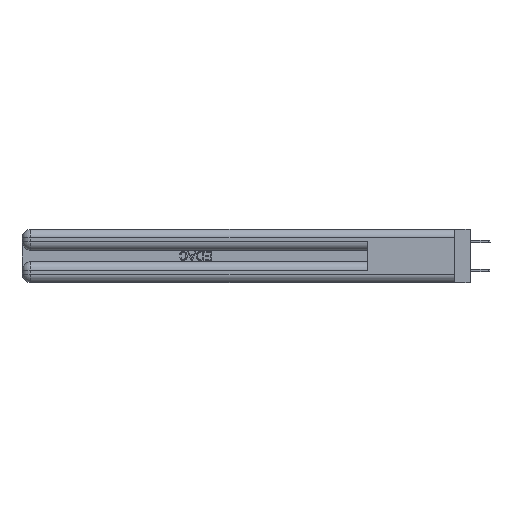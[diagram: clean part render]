
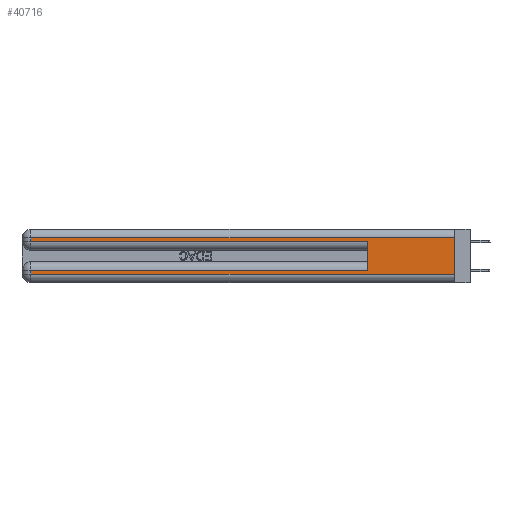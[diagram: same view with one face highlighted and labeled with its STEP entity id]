
A CAD part, left-side view. The second image highlights one B-rep face of the part: STEP entity #40716.
In plain terms, the highlighted planar face has unit normal (-1, 0, 0).
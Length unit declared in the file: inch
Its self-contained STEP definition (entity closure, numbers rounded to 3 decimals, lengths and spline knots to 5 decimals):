
#1308 = CARTESIAN_POINT ( 'NONE',  ( 0., 0., 0.37 ) ) ;
#1571 = DIRECTION ( 'NONE',  ( 0., -1., 0. ) ) ;
#2276 = AXIS2_PLACEMENT_3D ( 'NONE', #1308, #15779, #30198 ) ;
#2425 = VERTEX_POINT ( 'NONE', #5387 ) ;
#2899 = VERTEX_POINT ( 'NONE', #8666 ) ;
#4686 = VECTOR ( 'NONE', #23078, 39.37008 ) ;
#5306 = CARTESIAN_POINT ( 'NONE',  ( 0., 0.6, 0.085 ) ) ;
#5387 = CARTESIAN_POINT ( 'NONE',  ( 0., 2.94, 0.06 ) ) ;
#5488 = VECTOR ( 'NONE', #1571, 39.37008 ) ;
#7298 = EDGE_CURVE ( 'NONE', #46163, #21955, #8669, .T. ) ;
#7451 = EDGE_CURVE ( 'NONE', #21955, #2425, #9376, .T. ) ;
#8666 = CARTESIAN_POINT ( 'NONE',  ( 0., 2.94, 0.31 ) ) ;
#8669 = LINE ( 'NONE', #41094, #4686 ) ;
#9069 = DIRECTION ( 'NONE',  ( 0., 0., -1. ) ) ;
#9376 = LINE ( 'NONE', #13370, #44769 ) ;
#9484 = ORIENTED_EDGE ( 'NONE', *, *, #7298, .T. ) ;
#11022 = LINE ( 'NONE', #29865, #19572 ) ;
#11464 = DIRECTION ( 'NONE',  ( 0., -1., 0. ) ) ;
#12067 = CARTESIAN_POINT ( 'NONE',  ( 0., 0., 0.06 ) ) ;
#12344 = ORIENTED_EDGE ( 'NONE', *, *, #45141, .T. ) ;
#12583 = DIRECTION ( 'NONE',  ( 0., 1., 0. ) ) ;
#13263 = VERTEX_POINT ( 'NONE', #26310 ) ;
#13370 = CARTESIAN_POINT ( 'NONE',  ( 0., 2.94, 0.37 ) ) ;
#15779 = DIRECTION ( 'NONE',  ( 1., 0., 0. ) ) ;
#15793 = ORIENTED_EDGE ( 'NONE', *, *, #34491, .T. ) ;
#15811 = CARTESIAN_POINT ( 'NONE',  ( 0., 0.6, 0.145 ) ) ;
#16283 = DIRECTION ( 'NONE',  ( 0., 0., 1. ) ) ;
#16447 = DIRECTION ( 'NONE',  ( 0., 0., -1. ) ) ;
#19075 = ORIENTED_EDGE ( 'NONE', *, *, #24551, .F. ) ;
#19327 = FACE_OUTER_BOUND ( 'NONE', #39699, .T. ) ;
#19572 = VECTOR ( 'NONE', #29424, 39.37008 ) ;
#20062 = CARTESIAN_POINT ( 'NONE',  ( 0., 2.94, 0.085 ) ) ;
#21001 = VECTOR ( 'NONE', #12583, 39.37008 ) ;
#21955 = VERTEX_POINT ( 'NONE', #20062 ) ;
#22967 = VECTOR ( 'NONE', #11464, 39.37008 ) ;
#23078 = DIRECTION ( 'NONE',  ( 0., 1., 0. ) ) ;
#24154 = ORIENTED_EDGE ( 'NONE', *, *, #37795, .T. ) ;
#24551 = EDGE_CURVE ( 'NONE', #46163, #13263, #27652, .T. ) ;
#24935 = CARTESIAN_POINT ( 'NONE',  ( 0., 2.94, 0.285 ) ) ;
#25213 = VERTEX_POINT ( 'NONE', #24935 ) ;
#26141 = CARTESIAN_POINT ( 'NONE',  ( 0., 0., 0.06 ) ) ;
#26310 = CARTESIAN_POINT ( 'NONE',  ( 0., 0.6, 0.285 ) ) ;
#26341 = CARTESIAN_POINT ( 'NONE',  ( 0., 2.94, 0.37 ) ) ;
#27261 = LINE ( 'NONE', #26341, #36310 ) ;
#27652 = LINE ( 'NONE', #15811, #38621 ) ;
#29424 = DIRECTION ( 'NONE',  ( 0., 0., -1. ) ) ;
#29865 = CARTESIAN_POINT ( 'NONE',  ( 0., 0., 0.37 ) ) ;
#30198 = DIRECTION ( 'NONE',  ( 0., 0., -1. ) ) ;
#31731 = ORIENTED_EDGE ( 'NONE', *, *, #39120, .F. ) ;
#32503 = CARTESIAN_POINT ( 'NONE',  ( 0., 0., 0.285 ) ) ;
#32550 = VERTEX_POINT ( 'NONE', #26141 ) ;
#33764 = PLANE ( 'NONE',  #2276 ) ;
#34491 = EDGE_CURVE ( 'NONE', #39232, #2899, #38134, .T. ) ;
#36310 = VECTOR ( 'NONE', #9069, 39.37008 ) ;
#36511 = LINE ( 'NONE', #32503, #22967 ) ;
#37795 = EDGE_CURVE ( 'NONE', #2899, #25213, #27261, .T. ) ;
#38134 = LINE ( 'NONE', #45959, #21001 ) ;
#38621 = VECTOR ( 'NONE', #16283, 39.37008 ) ;
#39120 = EDGE_CURVE ( 'NONE', #39232, #32550, #11022, .T. ) ;
#39232 = VERTEX_POINT ( 'NONE', #41033 ) ;
#39699 = EDGE_LOOP ( 'NONE', ( #31731, #15793, #24154, #43012, #19075, #9484, #43278, #12344 ) ) ;
#40716 = ADVANCED_FACE ( 'NONE', ( #19327 ), #33764, .F. ) ;
#41033 = CARTESIAN_POINT ( 'NONE',  ( 0., 0., 0.31 ) ) ;
#41094 = CARTESIAN_POINT ( 'NONE',  ( 0., 0., 0.085 ) ) ;
#43012 = ORIENTED_EDGE ( 'NONE', *, *, #46488, .T. ) ;
#43278 = ORIENTED_EDGE ( 'NONE', *, *, #7451, .T. ) ;
#44038 = LINE ( 'NONE', #12067, #5488 ) ;
#44769 = VECTOR ( 'NONE', #16447, 39.37008 ) ;
#45141 = EDGE_CURVE ( 'NONE', #2425, #32550, #44038, .T. ) ;
#45959 = CARTESIAN_POINT ( 'NONE',  ( 0., 0., 0.31 ) ) ;
#46163 = VERTEX_POINT ( 'NONE', #5306 ) ;
#46488 = EDGE_CURVE ( 'NONE', #25213, #13263, #36511, .T. ) ;
